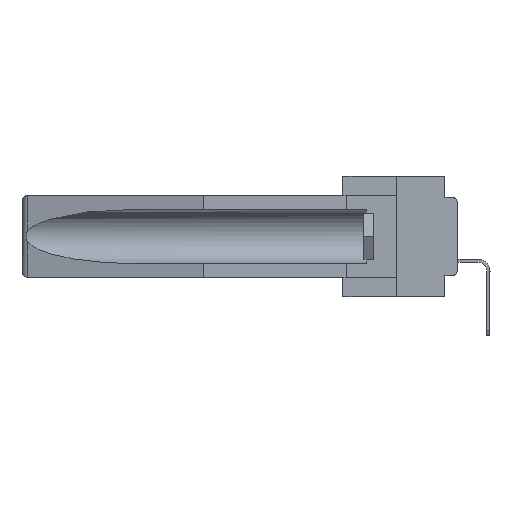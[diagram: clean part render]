
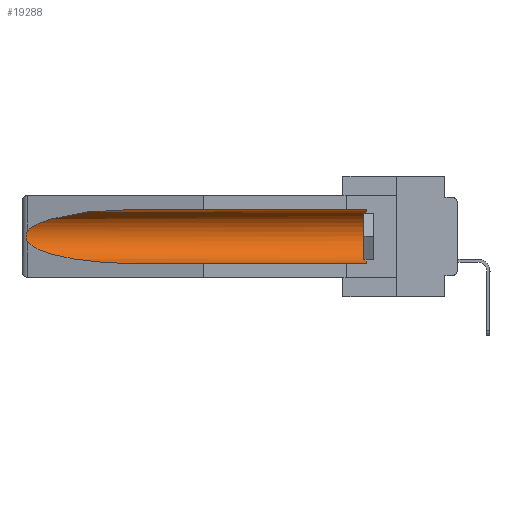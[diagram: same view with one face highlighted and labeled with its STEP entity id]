
A CAD part, left-side view. The second image highlights one B-rep face of the part: STEP entity #19288.
In plain terms, the highlighted cylindrical face has radius 2.857 mm (diameter 5.715 mm), a partial arc.
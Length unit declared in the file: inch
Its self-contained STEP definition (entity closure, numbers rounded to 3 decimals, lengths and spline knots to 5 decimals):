
#144 = CARTESIAN_POINT ( 'NONE',  ( 0.155, 1.07973, -0.284 ) ) ;
#467 =( BOUNDED_CURVE ( )  B_SPLINE_CURVE ( 3, ( #5679, #19064, #11231, #144 ),
 .UNSPECIFIED., .F., .F. ) 
 B_SPLINE_CURVE_WITH_KNOTS ( ( 4, 4 ),
 ( 0.1948, 1.5708 ),
 .UNSPECIFIED. ) 
 CURVE ( )  GEOMETRIC_REPRESENTATION_ITEM ( )  RATIONAL_B_SPLINE_CURVE ( ( 1., 0.848, 0.848, 1. ) ) 
 REPRESENTATION_ITEM ( '' )  );
#1673 = AXIS2_PLACEMENT_3D ( 'NONE', #21123, #31596, #13629 ) ;
#3463 = CARTESIAN_POINT ( 'NONE',  ( 0.2675, 1.53308, -0.16763 ) ) ;
#3500 = VERTEX_POINT ( 'NONE', #6408 ) ;
#4084 = CARTESIAN_POINT ( 'NONE',  ( 0.155, 0.126, -0.059 ) ) ;
#4638 = LINE ( 'NONE', #24401, #26521 ) ;
#5679 = CARTESIAN_POINT ( 'NONE',  ( 0.26537, 1.52718, -0.19328 ) ) ;
#6408 = CARTESIAN_POINT ( 'NONE',  ( 0.155, 0.126, -0.284 ) ) ;
#6460 = CARTESIAN_POINT ( 'NONE',  ( 0.2675, 1.53308, -0.17534 ) ) ;
#7851 = ORIENTED_EDGE ( 'NONE', *, *, #24683, .T. ) ;
#7975 = ORIENTED_EDGE ( 'NONE', *, *, #32386, .T. ) ;
#8331 = FACE_OUTER_BOUND ( 'NONE', #16071, .T. ) ;
#8523 = VERTEX_POINT ( 'NONE', #4084 ) ;
#8617 = DIRECTION ( 'NONE',  ( 0., 1., 0. ) ) ;
#9804 = VERTEX_POINT ( 'NONE', #32513 ) ;
#10152 = ORIENTED_EDGE ( 'NONE', *, *, #13501, .T. ) ;
#11231 = CARTESIAN_POINT ( 'NONE',  ( 0.21114, 1.30732, -0.284 ) ) ;
#11562 = CARTESIAN_POINT ( 'NONE',  ( 0.2673, 1.5327, -0.16383 ) ) ;
#11679 = CARTESIAN_POINT ( 'NONE',  ( 0.26654, 1.53092, -0.15636 ) ) ;
#12141 = B_SPLINE_CURVE_WITH_KNOTS ( 'NONE', 3,
 ( #22152, #24589, #11679, #11562, #3463, #6460, #14326, #25038, #19513, #30329 ),
 .UNSPECIFIED., .F., .F.,
 ( 4, 2, 2, 2, 4 ),
 ( 0., 0.00029, 0.00058, 0.00087, 0.00117 ),
 .UNSPECIFIED. ) ;
#13115 = CARTESIAN_POINT ( 'NONE',  ( 0.21114, 1.30732, -0.059 ) ) ;
#13341 = CARTESIAN_POINT ( 'NONE',  ( 0.25451, 1.48313, -0.09465 ) ) ;
#13501 = EDGE_CURVE ( 'NONE', #8523, #9804, #20379, .T. ) ;
#13629 = DIRECTION ( 'NONE',  ( 0., 0., 1. ) ) ;
#13918 = DIRECTION ( 'NONE',  ( 0., -1., 0. ) ) ;
#14326 = CARTESIAN_POINT ( 'NONE',  ( 0.2673, 1.53269, -0.17917 ) ) ;
#15770 = CARTESIAN_POINT ( 'NONE',  ( 0.26537, 1.52718, -0.14972 ) ) ;
#15836 = CIRCLE ( 'NONE', #33137, 0.1125 ) ;
#16071 = EDGE_LOOP ( 'NONE', ( #7975, #28436, #7851, #22140, #19045, #10152 ) ) ;
#16099 = CARTESIAN_POINT ( 'NONE',  ( 0.26537, 1.52718, -0.19328 ) ) ;
#16318 = EDGE_CURVE ( 'NONE', #20562, #18579, #12141, .T. ) ;
#16987 =( BOUNDED_CURVE ( )  B_SPLINE_CURVE ( 3, ( #23588, #13115, #13341, #15770 ),
 .UNSPECIFIED., .F., .F. ) 
 B_SPLINE_CURVE_WITH_KNOTS ( ( 4, 4 ),
 ( 4.71239, 6.08839 ),
 .UNSPECIFIED. ) 
 CURVE ( )  GEOMETRIC_REPRESENTATION_ITEM ( )  RATIONAL_B_SPLINE_CURVE ( ( 1., 0.848, 0.848, 1. ) ) 
 REPRESENTATION_ITEM ( '' )  );
#17307 = CARTESIAN_POINT ( 'NONE',  ( 0.155, 1.07973, -0.284 ) ) ;
#18233 = CARTESIAN_POINT ( 'NONE',  ( 0.155, -0.30754, -0.059 ) ) ;
#18320 = VERTEX_POINT ( 'NONE', #17307 ) ;
#18579 = VERTEX_POINT ( 'NONE', #16099 ) ;
#18665 = CYLINDRICAL_SURFACE ( 'NONE', #1673, 0.1125 ) ;
#18869 = CARTESIAN_POINT ( 'NONE',  ( 0.26537, 1.52718, -0.14972 ) ) ;
#19045 = ORIENTED_EDGE ( 'NONE', *, *, #32485, .T. ) ;
#19064 = CARTESIAN_POINT ( 'NONE',  ( 0.25451, 1.48313, -0.24835 ) ) ;
#19288 = ADVANCED_FACE ( 'NONE', ( #8331 ), #18665, .F. ) ;
#19513 = CARTESIAN_POINT ( 'NONE',  ( 0.26597, 1.5296, -0.19026 ) ) ;
#20379 = LINE ( 'NONE', #18233, #22820 ) ;
#20562 = VERTEX_POINT ( 'NONE', #18869 ) ;
#21123 = CARTESIAN_POINT ( 'NONE',  ( 0.155, -0.30754, -0.1715 ) ) ;
#22140 = ORIENTED_EDGE ( 'NONE', *, *, #23412, .F. ) ;
#22152 = CARTESIAN_POINT ( 'NONE',  ( 0.26537, 1.52718, -0.14972 ) ) ;
#22820 = VECTOR ( 'NONE', #31344, 39.37008 ) ;
#23412 = EDGE_CURVE ( 'NONE', #3500, #18320, #4638, .T. ) ;
#23588 = CARTESIAN_POINT ( 'NONE',  ( 0.155, 1.07973, -0.059 ) ) ;
#24401 = CARTESIAN_POINT ( 'NONE',  ( 0.155, -0.30754, -0.284 ) ) ;
#24589 = CARTESIAN_POINT ( 'NONE',  ( 0.26597, 1.52961, -0.15275 ) ) ;
#24683 = EDGE_CURVE ( 'NONE', #18579, #18320, #467, .T. ) ;
#25038 = CARTESIAN_POINT ( 'NONE',  ( 0.26655, 1.53094, -0.18657 ) ) ;
#26521 = VECTOR ( 'NONE', #8617, 39.37008 ) ;
#28436 = ORIENTED_EDGE ( 'NONE', *, *, #16318, .T. ) ;
#29690 = CARTESIAN_POINT ( 'NONE',  ( 0.155, 0.126, -0.1715 ) ) ;
#30329 = CARTESIAN_POINT ( 'NONE',  ( 0.26537, 1.52718, -0.19328 ) ) ;
#31344 = DIRECTION ( 'NONE',  ( 0., 1., 0. ) ) ;
#31596 = DIRECTION ( 'NONE',  ( 0., 1., 0. ) ) ;
#32386 = EDGE_CURVE ( 'NONE', #9804, #20562, #16987, .T. ) ;
#32485 = EDGE_CURVE ( 'NONE', #3500, #8523, #15836, .T. ) ;
#32513 = CARTESIAN_POINT ( 'NONE',  ( 0.155, 1.07973, -0.059 ) ) ;
#33004 = DIRECTION ( 'NONE',  ( 0., 0., 1. ) ) ;
#33137 = AXIS2_PLACEMENT_3D ( 'NONE', #29690, #13918, #33004 ) ;
